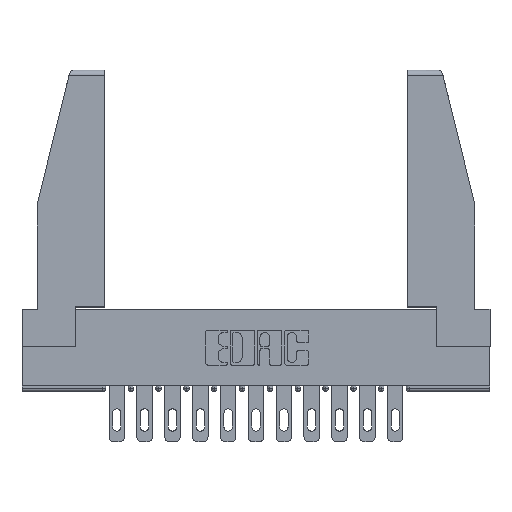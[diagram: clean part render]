
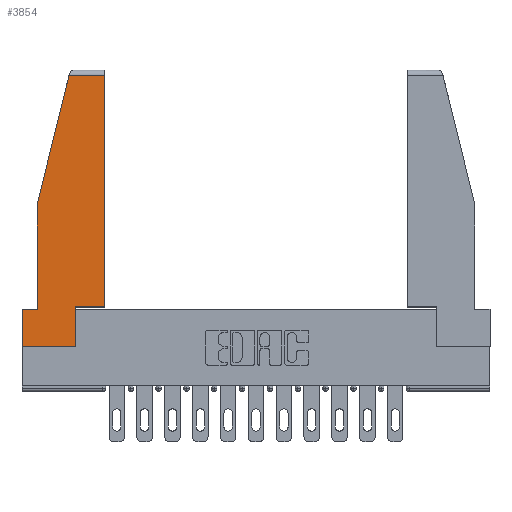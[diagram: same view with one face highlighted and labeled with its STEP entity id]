
A CAD part, top view. The second image highlights one B-rep face of the part: STEP entity #3854.
In plain terms, the highlighted planar face has unit normal (0, 0, 1).
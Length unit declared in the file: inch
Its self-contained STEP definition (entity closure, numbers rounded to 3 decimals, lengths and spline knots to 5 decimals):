
#14 = EDGE_CURVE ( 'NONE', #13752, #6221, #8718, .T. ) ;
#334 = VECTOR ( 'NONE', #10154, 39.37008 ) ;
#364 = ORIENTED_EDGE ( 'NONE', *, *, #16092, .T. ) ;
#805 = ORIENTED_EDGE ( 'NONE', *, *, #2750, .T. ) ;
#913 = CARTESIAN_POINT ( 'NONE',  ( 0.086, 0.21, 0. ) ) ;
#956 = LINE ( 'NONE', #1376, #10693 ) ;
#991 = LINE ( 'NONE', #5266, #7618 ) ;
#1315 = DIRECTION ( 'NONE',  ( 1., 0., 0. ) ) ;
#1376 = CARTESIAN_POINT ( 'NONE',  ( 0., 0.21, 0. ) ) ;
#1724 = EDGE_CURVE ( 'NONE', #5827, #8825, #10930, .T. ) ;
#2075 = ORIENTED_EDGE ( 'NONE', *, *, #16192, .T. ) ;
#2353 = EDGE_LOOP ( 'NONE', ( #3118, #16858, #2075, #3525, #12952, #7880, #364, #805, #13884 ) ) ;
#2465 = CARTESIAN_POINT ( 'NONE',  ( 0.271, 1.55, 0. ) ) ;
#2574 = DIRECTION ( 'NONE',  ( 0., 1., 0. ) ) ;
#2696 = VERTEX_POINT ( 'NONE', #4754 ) ;
#2750 = EDGE_CURVE ( 'NONE', #3616, #14082, #12671, .T. ) ;
#2812 = FACE_OUTER_BOUND ( 'NONE', #2353, .T. ) ;
#2855 = EDGE_CURVE ( 'NONE', #8825, #13752, #956, .T. ) ;
#3118 = ORIENTED_EDGE ( 'NONE', *, *, #6733, .T. ) ;
#3248 = LINE ( 'NONE', #8261, #16202 ) ;
#3525 = ORIENTED_EDGE ( 'NONE', *, *, #1724, .T. ) ;
#3616 = VERTEX_POINT ( 'NONE', #12477 ) ;
#3854 = ADVANCED_FACE ( 'NONE', ( #2812 ), #7847, .T. ) ;
#4711 = CARTESIAN_POINT ( 'NONE',  ( 0.086, 0.8, 0. ) ) ;
#4754 = CARTESIAN_POINT ( 'NONE',  ( 0.461, 0.223, 0. ) ) ;
#4889 = DIRECTION ( 'NONE',  ( 1., 0., 0. ) ) ;
#5223 = AXIS2_PLACEMENT_3D ( 'NONE', #7011, #11040, #12678 ) ;
#5266 = CARTESIAN_POINT ( 'NONE',  ( 0.297, 0.223, 0. ) ) ;
#5318 = CARTESIAN_POINT ( 'NONE',  ( 0., 0.21, 0. ) ) ;
#5489 = VECTOR ( 'NONE', #2574, 39.37008 ) ;
#5604 = DIRECTION ( 'NONE',  ( -1., 0., 0. ) ) ;
#5737 = EDGE_CURVE ( 'NONE', #7758, #10706, #3248, .T. ) ;
#5827 = VERTEX_POINT ( 'NONE', #4711 ) ;
#6221 = VERTEX_POINT ( 'NONE', #6685 ) ;
#6413 = DIRECTION ( 'NONE',  ( -1., 0., 0. ) ) ;
#6685 = CARTESIAN_POINT ( 'NONE',  ( 0., 0., 0. ) ) ;
#6733 = EDGE_CURVE ( 'NONE', #2696, #7758, #12421, .T. ) ;
#7011 = CARTESIAN_POINT ( 'NONE',  ( 0., 0., 0. ) ) ;
#7618 = VECTOR ( 'NONE', #1315, 39.37008 ) ;
#7758 = VERTEX_POINT ( 'NONE', #9978 ) ;
#7847 = PLANE ( 'NONE',  #5223 ) ;
#7880 = ORIENTED_EDGE ( 'NONE', *, *, #14, .T. ) ;
#8170 = VECTOR ( 'NONE', #4889, 39.37008 ) ;
#8261 = CARTESIAN_POINT ( 'NONE',  ( 0., 1.52, 0. ) ) ;
#8300 = VECTOR ( 'NONE', #10285, 39.37008 ) ;
#8718 = LINE ( 'NONE', #5318, #8300 ) ;
#8825 = VERTEX_POINT ( 'NONE', #913 ) ;
#8850 = VECTOR ( 'NONE', #12315, 39.37008 ) ;
#9626 = CARTESIAN_POINT ( 'NONE',  ( 0.086, 0.8, 0. ) ) ;
#9875 = CARTESIAN_POINT ( 'NONE',  ( 0.297, 0.223, 0. ) ) ;
#9978 = CARTESIAN_POINT ( 'NONE',  ( 0.461, 1.52, 0. ) ) ;
#10154 = DIRECTION ( 'NONE',  ( 0., -1., 0. ) ) ;
#10285 = DIRECTION ( 'NONE',  ( 0., -1., 0. ) ) ;
#10693 = VECTOR ( 'NONE', #6413, 39.37008 ) ;
#10706 = VERTEX_POINT ( 'NONE', #13037 ) ;
#10930 = LINE ( 'NONE', #9626, #334 ) ;
#11025 = EDGE_CURVE ( 'NONE', #14082, #2696, #991, .T. ) ;
#11040 = DIRECTION ( 'NONE',  ( 0., 0., 1. ) ) ;
#11222 = LINE ( 'NONE', #13935, #8170 ) ;
#12315 = DIRECTION ( 'NONE',  ( 0., 1., 0. ) ) ;
#12421 = LINE ( 'NONE', #14262, #5489 ) ;
#12477 = CARTESIAN_POINT ( 'NONE',  ( 0.297, 0., 0. ) ) ;
#12671 = LINE ( 'NONE', #16820, #8850 ) ;
#12678 = DIRECTION ( 'NONE',  ( 1., 0., 0. ) ) ;
#12933 = DIRECTION ( 'NONE',  ( -0.239, -0.971, 0. ) ) ;
#12952 = ORIENTED_EDGE ( 'NONE', *, *, #2855, .T. ) ;
#13037 = CARTESIAN_POINT ( 'NONE',  ( 0.2636, 1.52, 0. ) ) ;
#13401 = VECTOR ( 'NONE', #12933, 39.37008 ) ;
#13752 = VERTEX_POINT ( 'NONE', #16579 ) ;
#13884 = ORIENTED_EDGE ( 'NONE', *, *, #11025, .T. ) ;
#13935 = CARTESIAN_POINT ( 'NONE',  ( 0., 0., 0. ) ) ;
#14082 = VERTEX_POINT ( 'NONE', #9875 ) ;
#14262 = CARTESIAN_POINT ( 'NONE',  ( 0.461, 0.223, 0. ) ) ;
#16092 = EDGE_CURVE ( 'NONE', #6221, #3616, #11222, .T. ) ;
#16192 = EDGE_CURVE ( 'NONE', #10706, #5827, #16743, .T. ) ;
#16202 = VECTOR ( 'NONE', #5604, 39.37008 ) ;
#16579 = CARTESIAN_POINT ( 'NONE',  ( 0., 0.21, 0. ) ) ;
#16743 = LINE ( 'NONE', #2465, #13401 ) ;
#16820 = CARTESIAN_POINT ( 'NONE',  ( 0.297, 0., 0. ) ) ;
#16858 = ORIENTED_EDGE ( 'NONE', *, *, #5737, .T. ) ;
